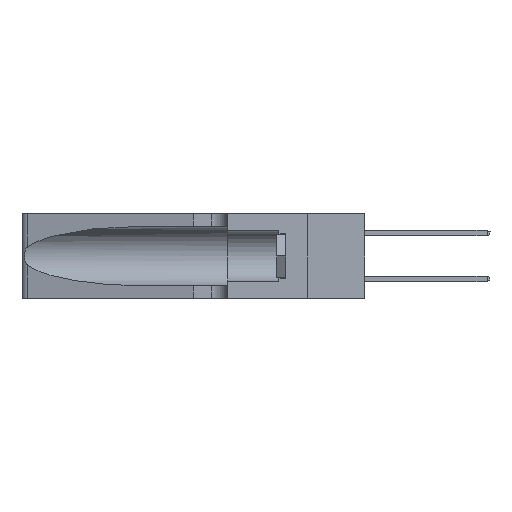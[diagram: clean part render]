
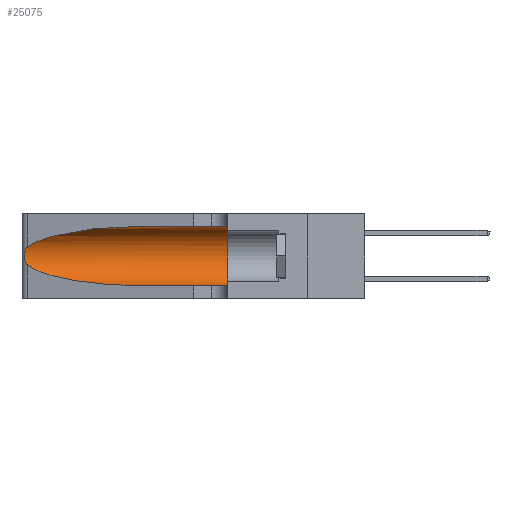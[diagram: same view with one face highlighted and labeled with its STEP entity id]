
A CAD part, left-side view. The second image highlights one B-rep face of the part: STEP entity #25075.
In plain terms, the highlighted cylindrical face has radius 3.308 mm (diameter 6.617 mm), a partial arc.
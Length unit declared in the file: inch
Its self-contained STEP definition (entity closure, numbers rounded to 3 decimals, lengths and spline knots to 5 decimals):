
#904 = CARTESIAN_POINT ( 'NONE',  ( 0.25487, 1.22718, 0.22369 ) ) ;
#1446 = DIRECTION ( 'NONE',  ( 0., -1., 0. ) ) ;
#1841 = DIRECTION ( 'NONE',  ( 0., 0., -1. ) ) ;
#2027 = DIRECTION ( 'NONE',  ( 0., -1., 0. ) ) ;
#2276 = VERTEX_POINT ( 'NONE', #2365 ) ;
#2365 = CARTESIAN_POINT ( 'NONE',  ( 0.25487, 1.22718, 0.14631 ) ) ;
#3947 = CARTESIAN_POINT ( 'NONE',  ( 0.2373, 1.15595, 0.08982 ) ) ;
#5051 = CARTESIAN_POINT ( 'NONE',  ( 0.1305, 1.61858, 0.31525 ) ) ;
#6021 = CARTESIAN_POINT ( 'NONE',  ( 0.26075, 1.23896, 0.19203 ) ) ;
#7304 = LINE ( 'NONE', #20741, #32132 ) ;
#7366 = CARTESIAN_POINT ( 'NONE',  ( 0.2373, 1.15595, 0.28018 ) ) ;
#9211 = CARTESIAN_POINT ( 'NONE',  ( 0.26017, 1.23833, 0.17102 ) ) ;
#10280 = CARTESIAN_POINT ( 'NONE',  ( 0.1305, 0.72297, 0.31525 ) ) ;
#10331 = VECTOR ( 'NONE', #17529, 39.37008 ) ;
#10812 = CARTESIAN_POINT ( 'NONE',  ( 0.25487, 1.22718, 0.22369 ) ) ;
#11118 = EDGE_CURVE ( 'NONE', #11366, #39333, #18556, .T. ) ;
#11366 = VERTEX_POINT ( 'NONE', #28790 ) ;
#12406 = CARTESIAN_POINT ( 'NONE',  ( 0.25856, 1.23593, 0.16098 ) ) ;
#13466 = CARTESIAN_POINT ( 'NONE',  ( 0.18966, 0.96281, 0.31525 ) ) ;
#13692 = EDGE_CURVE ( 'NONE', #36136, #36837, #7304, .T. ) ;
#15615 = CARTESIAN_POINT ( 'NONE',  ( 0.25639, 1.23186, 0.15144 ) ) ;
#15804 = ORIENTED_EDGE ( 'NONE', *, *, #23227, .T. ) ;
#16015 = CARTESIAN_POINT ( 'NONE',  ( 0.25854, 1.2359, 0.20912 ) ) ;
#16448 = CARTESIAN_POINT ( 'NONE',  ( 0.18966, 0.96281, 0.05475 ) ) ;
#16540 = ORIENTED_EDGE ( 'NONE', *, *, #24542, .F. ) ;
#17047 = ORIENTED_EDGE ( 'NONE', *, *, #11118, .T. ) ;
#17529 = DIRECTION ( 'NONE',  ( 0., -1., 0. ) ) ;
#18370 = ORIENTED_EDGE ( 'NONE', *, *, #38408, .T. ) ;
#18556 =( BOUNDED_CURVE ( )  B_SPLINE_CURVE ( 3, ( #10280, #13466, #7366, #904 ),
 .UNSPECIFIED., .F., .F. ) 
 B_SPLINE_CURVE_WITH_KNOTS ( ( 4, 4 ),
 ( 1.5708, 2.84003 ),
 .UNSPECIFIED. ) 
 CURVE ( )  GEOMETRIC_REPRESENTATION_ITEM ( )  RATIONAL_B_SPLINE_CURVE ( ( 1., 0.87, 0.87, 1. ) ) 
 REPRESENTATION_ITEM ( '' )  );
#18727 = CARTESIAN_POINT ( 'NONE',  ( 0.1305, 0.35, 0.185 ) ) ;
#18797 = CARTESIAN_POINT ( 'NONE',  ( 0.25555, 1.22993, 0.14849 ) ) ;
#20741 = CARTESIAN_POINT ( 'NONE',  ( 0.1305, 1.61858, 0.05475 ) ) ;
#21266 = CARTESIAN_POINT ( 'NONE',  ( 0.1305, 0.35, 0.31525 ) ) ;
#21870 = AXIS2_PLACEMENT_3D ( 'NONE', #29676, #1446, #1841 ) ;
#22446 = CARTESIAN_POINT ( 'NONE',  ( 0.1305, 0.72297, 0.05475 ) ) ;
#22964 = CARTESIAN_POINT ( 'NONE',  ( 0.25487, 1.22718, 0.14631 ) ) ;
#23227 = EDGE_CURVE ( 'NONE', #2276, #36136, #33320, .T. ) ;
#23600 = EDGE_CURVE ( 'NONE', #28424, #36837, #24791, .T. ) ;
#24542 = EDGE_CURVE ( 'NONE', #11366, #28424, #36643, .T. ) ;
#24791 = CIRCLE ( 'NONE', #28485, 0.13025 ) ;
#25075 = ADVANCED_FACE ( 'NONE', ( #26622 ), #30145, .F. ) ;
#25283 = CARTESIAN_POINT ( 'NONE',  ( 0.1305, 0.35, 0.05475 ) ) ;
#26622 = FACE_OUTER_BOUND ( 'NONE', #30186, .T. ) ;
#27970 = DIRECTION ( 'NONE',  ( 0., 1., 0. ) ) ;
#28176 = CARTESIAN_POINT ( 'NONE',  ( 0.26075, 1.23896, 0.178 ) ) ;
#28240 = ORIENTED_EDGE ( 'NONE', *, *, #13692, .T. ) ;
#28424 = VERTEX_POINT ( 'NONE', #21266 ) ;
#28485 = AXIS2_PLACEMENT_3D ( 'NONE', #18727, #27970, #37825 ) ;
#28790 = CARTESIAN_POINT ( 'NONE',  ( 0.1305, 0.72297, 0.31525 ) ) ;
#28891 = CARTESIAN_POINT ( 'NONE',  ( 0.1305, 0.72297, 0.05475 ) ) ;
#29593 = ORIENTED_EDGE ( 'NONE', *, *, #23600, .F. ) ;
#29676 = CARTESIAN_POINT ( 'NONE',  ( 0.1305, 1.61858, 0.185 ) ) ;
#30145 = CYLINDRICAL_SURFACE ( 'NONE', #21870, 0.13025 ) ;
#30186 = EDGE_LOOP ( 'NONE', ( #17047, #18370, #15804, #28240, #29593, #16540 ) ) ;
#31365 = CARTESIAN_POINT ( 'NONE',  ( 0.25639, 1.23184, 0.21858 ) ) ;
#31791 = CARTESIAN_POINT ( 'NONE',  ( 0.25555, 1.22994, 0.2215 ) ) ;
#32132 = VECTOR ( 'NONE', #2027, 39.37008 ) ;
#33320 =( BOUNDED_CURVE ( )  B_SPLINE_CURVE ( 3, ( #22964, #3947, #16448, #28891 ),
 .UNSPECIFIED., .F., .T. ) 
 B_SPLINE_CURVE_WITH_KNOTS ( ( 4, 4 ),
 ( 3.44316, 4.71239 ),
 .UNSPECIFIED. ) 
 CURVE ( )  GEOMETRIC_REPRESENTATION_ITEM ( )  RATIONAL_B_SPLINE_CURVE ( ( 1., 0.87, 0.87, 1. ) ) 
 REPRESENTATION_ITEM ( '' )  );
#34612 = CARTESIAN_POINT ( 'NONE',  ( 0.25789, 1.23486, 0.15765 ) ) ;
#34879 = CARTESIAN_POINT ( 'NONE',  ( 0.25487, 1.22718, 0.22369 ) ) ;
#35017 = CARTESIAN_POINT ( 'NONE',  ( 0.25787, 1.23484, 0.2124 ) ) ;
#36136 = VERTEX_POINT ( 'NONE', #22446 ) ;
#36643 = LINE ( 'NONE', #5051, #10331 ) ;
#36837 = VERTEX_POINT ( 'NONE', #25283 ) ;
#37090 = B_SPLINE_CURVE_WITH_KNOTS ( 'NONE', 3,
 ( #34879, #31791, #31365, #35017, #16015, #40792, #6021, #28176, #9211, #12406, #34612, #15615, #18797, #40946 ),
 .UNSPECIFIED., .F., .F.,
 ( 4, 2, 2, 2, 2, 2, 4 ),
 ( 0., 0.00027, 0.00053, 0.00107, 0.0016, 0.00187, 0.00214 ),
 .UNSPECIFIED. ) ;
#37825 = DIRECTION ( 'NONE',  ( 0., 0., 1. ) ) ;
#38408 = EDGE_CURVE ( 'NONE', #39333, #2276, #37090, .T. ) ;
#39333 = VERTEX_POINT ( 'NONE', #10812 ) ;
#40792 = CARTESIAN_POINT ( 'NONE',  ( 0.26018, 1.23835, 0.19895 ) ) ;
#40946 = CARTESIAN_POINT ( 'NONE',  ( 0.25487, 1.22718, 0.14631 ) ) ;
